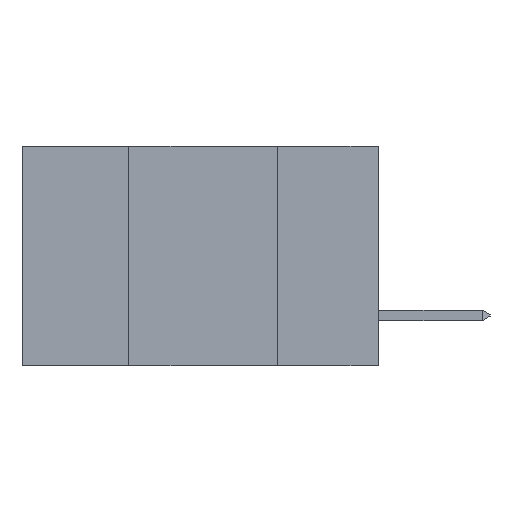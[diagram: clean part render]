
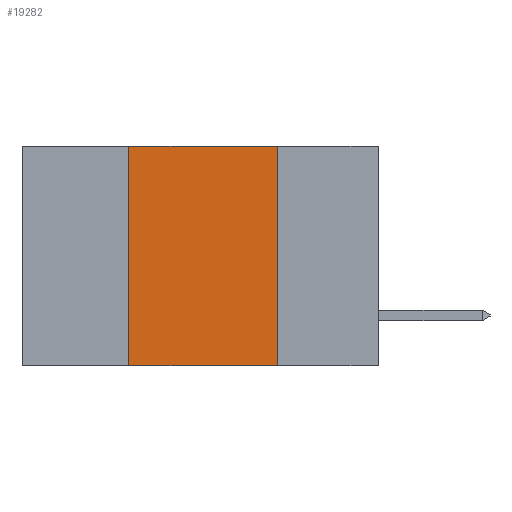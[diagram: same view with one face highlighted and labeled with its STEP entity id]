
A CAD part, left-side view. The second image highlights one B-rep face of the part: STEP entity #19282.
In plain terms, the highlighted planar face has unit normal (-1, 0, 0).
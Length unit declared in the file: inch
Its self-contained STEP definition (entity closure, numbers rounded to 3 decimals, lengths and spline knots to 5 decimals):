
#1116 = PLANE ( 'NONE',  #20947 ) ;
#1185 = DIRECTION ( 'NONE',  ( 1., 0., 0. ) ) ;
#1221 = CARTESIAN_POINT ( 'NONE',  ( 0., 0.6, 0. ) ) ;
#1469 = EDGE_LOOP ( 'NONE', ( #15433, #17945, #6410, #11393 ) ) ;
#1506 = CARTESIAN_POINT ( 'NONE',  ( 0., 0.17, -0.37 ) ) ;
#1744 = EDGE_CURVE ( 'NONE', #15008, #13173, #9138, .T. ) ;
#2663 = VERTEX_POINT ( 'NONE', #10651 ) ;
#3022 = LINE ( 'NONE', #4669, #11907 ) ;
#3194 = DIRECTION ( 'NONE',  ( 0., 0., -1. ) ) ;
#4009 = LINE ( 'NONE', #1221, #7962 ) ;
#4669 = CARTESIAN_POINT ( 'NONE',  ( 0., 0.42, -0.37 ) ) ;
#4696 = VECTOR ( 'NONE', #4887, 39.37008 ) ;
#4887 = DIRECTION ( 'NONE',  ( 0., -1., 0. ) ) ;
#6410 = ORIENTED_EDGE ( 'NONE', *, *, #12228, .F. ) ;
#7135 = CARTESIAN_POINT ( 'NONE',  ( 0., 0.6, -0.37 ) ) ;
#7188 = CARTESIAN_POINT ( 'NONE',  ( 0., 0.17, -0.37 ) ) ;
#7791 = EDGE_CURVE ( 'NONE', #2663, #13173, #8564, .T. ) ;
#7962 = VECTOR ( 'NONE', #12883, 39.37008 ) ;
#8564 = LINE ( 'NONE', #1506, #16744 ) ;
#9138 = LINE ( 'NONE', #7135, #4696 ) ;
#10029 = EDGE_CURVE ( 'NONE', #18631, #2663, #4009, .T. ) ;
#10651 = CARTESIAN_POINT ( 'NONE',  ( 0., 0.17, 0. ) ) ;
#11263 = CARTESIAN_POINT ( 'NONE',  ( 0., 0.6, 0. ) ) ;
#11393 = ORIENTED_EDGE ( 'NONE', *, *, #1744, .T. ) ;
#11907 = VECTOR ( 'NONE', #12988, 39.37008 ) ;
#12228 = EDGE_CURVE ( 'NONE', #15008, #18631, #3022, .T. ) ;
#12399 = FACE_OUTER_BOUND ( 'NONE', #1469, .T. ) ;
#12851 = DIRECTION ( 'NONE',  ( 0., 0., -1. ) ) ;
#12883 = DIRECTION ( 'NONE',  ( 0., -1., 0. ) ) ;
#12988 = DIRECTION ( 'NONE',  ( 0., 0., 1. ) ) ;
#13173 = VERTEX_POINT ( 'NONE', #7188 ) ;
#15008 = VERTEX_POINT ( 'NONE', #16397 ) ;
#15433 = ORIENTED_EDGE ( 'NONE', *, *, #7791, .F. ) ;
#16397 = CARTESIAN_POINT ( 'NONE',  ( 0., 0.42, -0.37 ) ) ;
#16744 = VECTOR ( 'NONE', #3194, 39.37008 ) ;
#17945 = ORIENTED_EDGE ( 'NONE', *, *, #10029, .F. ) ;
#18631 = VERTEX_POINT ( 'NONE', #19302 ) ;
#19282 = ADVANCED_FACE ( 'NONE', ( #12399 ), #1116, .F. ) ;
#19302 = CARTESIAN_POINT ( 'NONE',  ( 0., 0.42, 0. ) ) ;
#20947 = AXIS2_PLACEMENT_3D ( 'NONE', #11263, #1185, #12851 ) ;
